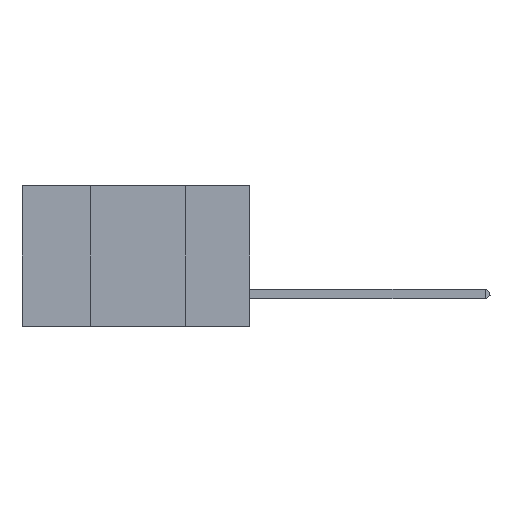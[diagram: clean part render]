
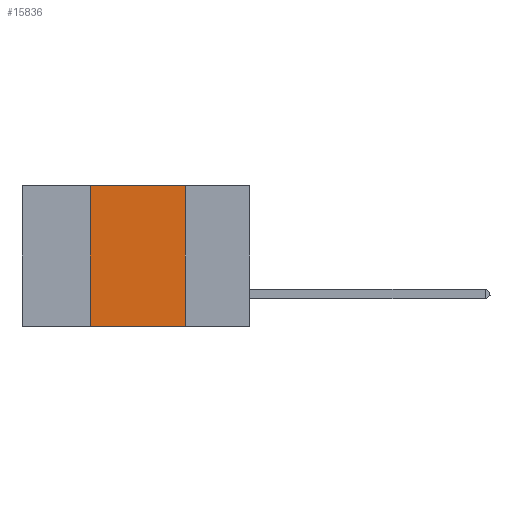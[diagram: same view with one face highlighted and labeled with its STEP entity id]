
A CAD part, left-side view. The second image highlights one B-rep face of the part: STEP entity #15836.
In plain terms, the highlighted planar face has unit normal (-1, 0, 0).
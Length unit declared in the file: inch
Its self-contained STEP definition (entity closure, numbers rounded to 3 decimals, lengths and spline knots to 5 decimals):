
#560 = ORIENTED_EDGE ( 'NONE', *, *, #31450, .T. ) ;
#2622 = ORIENTED_EDGE ( 'NONE', *, *, #30895, .F. ) ;
#3727 = VERTEX_POINT ( 'NONE', #45906 ) ;
#5369 = EDGE_CURVE ( 'NONE', #46618, #27880, #27473, .T. ) ;
#6975 = EDGE_LOOP ( 'NONE', ( #36687, #29430, #2622, #560 ) ) ;
#7682 = DIRECTION ( 'NONE',  ( 0., -1., 0. ) ) ;
#8269 = FACE_OUTER_BOUND ( 'NONE', #6975, .T. ) ;
#10140 = LINE ( 'NONE', #27611, #24694 ) ;
#10539 = VECTOR ( 'NONE', #10788, 39.37008 ) ;
#10788 = DIRECTION ( 'NONE',  ( 0., 0., 1. ) ) ;
#11026 = DIRECTION ( 'NONE',  ( 1., 0., 0. ) ) ;
#11106 = VERTEX_POINT ( 'NONE', #48401 ) ;
#11192 = CARTESIAN_POINT ( 'NONE',  ( 0., 0.6, 0. ) ) ;
#11463 = CARTESIAN_POINT ( 'NONE',  ( 0., 0.42, 0. ) ) ;
#13470 = VECTOR ( 'NONE', #7682, 39.37008 ) ;
#14137 = DIRECTION ( 'NONE',  ( 0., -1., 0. ) ) ;
#15836 = ADVANCED_FACE ( 'NONE', ( #8269 ), #18799, .F. ) ;
#18799 = PLANE ( 'NONE',  #37669 ) ;
#24694 = VECTOR ( 'NONE', #39044, 39.37008 ) ;
#24995 = EDGE_CURVE ( 'NONE', #27880, #3727, #10140, .T. ) ;
#27473 = LINE ( 'NONE', #30971, #13470 ) ;
#27611 = CARTESIAN_POINT ( 'NONE',  ( 0., 0.17, 0. ) ) ;
#27880 = VERTEX_POINT ( 'NONE', #48579 ) ;
#29430 = ORIENTED_EDGE ( 'NONE', *, *, #5369, .F. ) ;
#29614 = CARTESIAN_POINT ( 'NONE',  ( 0., 0.6, -0.37 ) ) ;
#30895 = EDGE_CURVE ( 'NONE', #11106, #46618, #41591, .T. ) ;
#30971 = CARTESIAN_POINT ( 'NONE',  ( 0., 0.6, 0. ) ) ;
#31450 = EDGE_CURVE ( 'NONE', #11106, #3727, #37315, .T. ) ;
#32388 = VECTOR ( 'NONE', #14137, 39.37008 ) ;
#32748 = CARTESIAN_POINT ( 'NONE',  ( 0., 0.42, 0. ) ) ;
#36687 = ORIENTED_EDGE ( 'NONE', *, *, #24995, .F. ) ;
#37315 = LINE ( 'NONE', #29614, #32388 ) ;
#37669 = AXIS2_PLACEMENT_3D ( 'NONE', #11192, #11026, #38439 ) ;
#38439 = DIRECTION ( 'NONE',  ( 0., 0., -1. ) ) ;
#39044 = DIRECTION ( 'NONE',  ( 0., 0., -1. ) ) ;
#41591 = LINE ( 'NONE', #11463, #10539 ) ;
#45906 = CARTESIAN_POINT ( 'NONE',  ( 0., 0.17, -0.37 ) ) ;
#46618 = VERTEX_POINT ( 'NONE', #32748 ) ;
#48401 = CARTESIAN_POINT ( 'NONE',  ( 0., 0.42, -0.37 ) ) ;
#48579 = CARTESIAN_POINT ( 'NONE',  ( 0., 0.17, 0. ) ) ;
